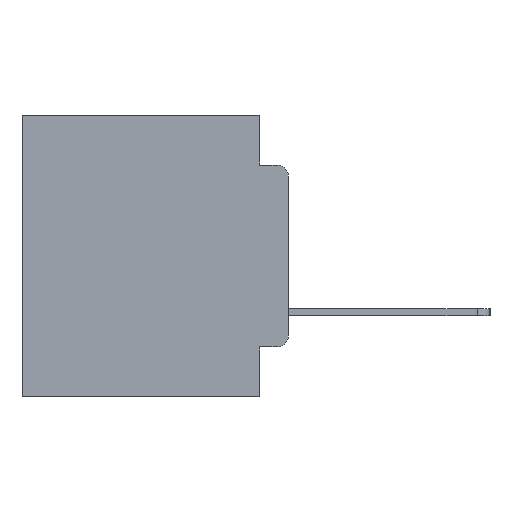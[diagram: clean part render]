
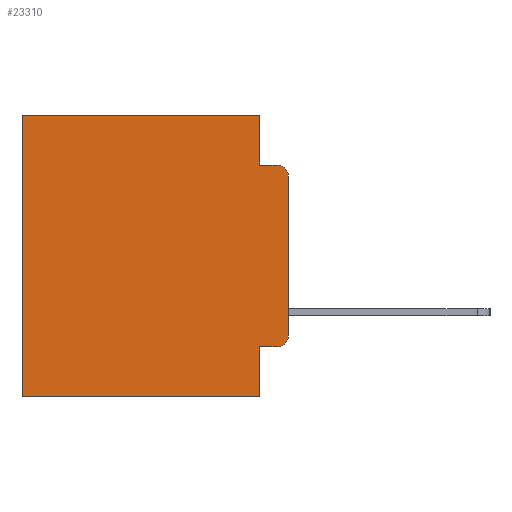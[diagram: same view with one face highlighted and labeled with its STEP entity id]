
A CAD part, left-side view. The second image highlights one B-rep face of the part: STEP entity #23310.
In plain terms, the highlighted planar face has unit normal (-1, 0, 0).
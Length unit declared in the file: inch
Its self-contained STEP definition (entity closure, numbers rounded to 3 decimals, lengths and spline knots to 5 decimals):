
#515 = VERTEX_POINT ( 'NONE', #2719 ) ;
#651 = CARTESIAN_POINT ( 'NONE',  ( 0.298, 0., -0.5 ) ) ;
#841 = EDGE_CURVE ( 'NONE', #9503, #11360, #6583, .T. ) ;
#1132 = CARTESIAN_POINT ( 'NONE',  ( 0.298, 0., -0.1085 ) ) ;
#2231 = ORIENTED_EDGE ( 'NONE', *, *, #3805, .T. ) ;
#2338 = EDGE_CURVE ( 'NONE', #9503, #2474, #14834, .T. ) ;
#2396 = CARTESIAN_POINT ( 'NONE',  ( 0.298, 0.473, 0. ) ) ;
#2474 = VERTEX_POINT ( 'NONE', #25600 ) ;
#2607 = CARTESIAN_POINT ( 'NONE',  ( 0.298, 0.02, -0.4115 ) ) ;
#2719 = CARTESIAN_POINT ( 'NONE',  ( 0.298, 0., -0.3915 ) ) ;
#2882 = DIRECTION ( 'NONE',  ( 0., 1., 0. ) ) ;
#3184 = VECTOR ( 'NONE', #17346, 39.37008 ) ;
#3805 = EDGE_CURVE ( 'NONE', #10068, #22903, #26704, .T. ) ;
#4160 = CARTESIAN_POINT ( 'NONE',  ( 0.298, 0., 0. ) ) ;
#4231 = LINE ( 'NONE', #8082, #25901 ) ;
#4337 = LINE ( 'NONE', #25617, #26009 ) ;
#5426 = AXIS2_PLACEMENT_3D ( 'NONE', #4160, #23135, #10637 ) ;
#5854 = DIRECTION ( 'NONE',  ( 0., -1., 0. ) ) ;
#6113 = DIRECTION ( 'NONE',  ( 0., 0., -1. ) ) ;
#6281 = AXIS2_PLACEMENT_3D ( 'NONE', #19932, #7382, #22053 ) ;
#6313 = DIRECTION ( 'NONE',  ( 0., 0., -1. ) ) ;
#6583 = LINE ( 'NONE', #18797, #17134 ) ;
#6631 = CARTESIAN_POINT ( 'NONE',  ( 0.298, 0.051, -0.4115 ) ) ;
#6739 = EDGE_CURVE ( 'NONE', #25268, #25956, #12794, .T. ) ;
#7143 = VECTOR ( 'NONE', #24099, 39.37008 ) ;
#7382 = DIRECTION ( 'NONE',  ( -1., 0., 0. ) ) ;
#7748 = FACE_OUTER_BOUND ( 'NONE', #19220, .T. ) ;
#8082 = CARTESIAN_POINT ( 'NONE',  ( 0.298, 0., 0. ) ) ;
#8190 = EDGE_CURVE ( 'NONE', #25956, #24409, #4337, .T. ) ;
#8377 = ORIENTED_EDGE ( 'NONE', *, *, #9602, .T. ) ;
#9370 = ORIENTED_EDGE ( 'NONE', *, *, #841, .T. ) ;
#9503 = VERTEX_POINT ( 'NONE', #6631 ) ;
#9602 = EDGE_CURVE ( 'NONE', #19210, #24409, #12282, .T. ) ;
#10068 = VERTEX_POINT ( 'NONE', #2396 ) ;
#10109 = VECTOR ( 'NONE', #6113, 39.37008 ) ;
#10637 = DIRECTION ( 'NONE',  ( 0., 0., -1. ) ) ;
#11360 = VERTEX_POINT ( 'NONE', #2607 ) ;
#12282 = CIRCLE ( 'NONE', #6281, 0.02 ) ;
#12420 = EDGE_CURVE ( 'NONE', #19210, #515, #4231, .T. ) ;
#12647 = EDGE_CURVE ( 'NONE', #25268, #10068, #20061, .T. ) ;
#12650 = CARTESIAN_POINT ( 'NONE',  ( 0.298, 0.02, -0.3915 ) ) ;
#12675 = PLANE ( 'NONE',  #5426 ) ;
#12794 = LINE ( 'NONE', #22020, #7143 ) ;
#13660 = ORIENTED_EDGE ( 'NONE', *, *, #2338, .F. ) ;
#14770 = DIRECTION ( 'NONE',  ( 0., 0., -1. ) ) ;
#14834 = LINE ( 'NONE', #15004, #19034 ) ;
#15004 = CARTESIAN_POINT ( 'NONE',  ( 0.298, 0.051, 0. ) ) ;
#15262 = CARTESIAN_POINT ( 'NONE',  ( 0.298, 0., 0. ) ) ;
#15452 = CARTESIAN_POINT ( 'NONE',  ( 0.298, 0.473, -0.5 ) ) ;
#15798 = CARTESIAN_POINT ( 'NONE',  ( 0.298, 0.051, -0.0885 ) ) ;
#16183 = DIRECTION ( 'NONE',  ( 0., -1., 0. ) ) ;
#16511 = EDGE_CURVE ( 'NONE', #2474, #22903, #26353, .T. ) ;
#16595 = ORIENTED_EDGE ( 'NONE', *, *, #8190, .F. ) ;
#16808 = CARTESIAN_POINT ( 'NONE',  ( 0.298, 0.473, 0. ) ) ;
#17134 = VECTOR ( 'NONE', #5854, 39.37008 ) ;
#17346 = DIRECTION ( 'NONE',  ( 0., 1., 0. ) ) ;
#17883 = ORIENTED_EDGE ( 'NONE', *, *, #12647, .T. ) ;
#18680 = AXIS2_PLACEMENT_3D ( 'NONE', #12650, #27131, #14770 ) ;
#18797 = CARTESIAN_POINT ( 'NONE',  ( 0.298, 0.051, -0.4115 ) ) ;
#19034 = VECTOR ( 'NONE', #6313, 39.37008 ) ;
#19167 = ORIENTED_EDGE ( 'NONE', *, *, #16511, .F. ) ;
#19210 = VERTEX_POINT ( 'NONE', #1132 ) ;
#19220 = EDGE_LOOP ( 'NONE', ( #26283, #8377, #16595, #23405, #17883, #2231, #19167, #13660, #9370, #20463 ) ) ;
#19316 = CARTESIAN_POINT ( 'NONE',  ( 0.298, 0.051, 0. ) ) ;
#19932 = CARTESIAN_POINT ( 'NONE',  ( 0.298, 0.02, -0.1085 ) ) ;
#20061 = LINE ( 'NONE', #15262, #3184 ) ;
#20463 = ORIENTED_EDGE ( 'NONE', *, *, #26836, .T. ) ;
#20631 = CARTESIAN_POINT ( 'NONE',  ( 0.298, 0.02, -0.0885 ) ) ;
#20766 = CIRCLE ( 'NONE', #18680, 0.02 ) ;
#22020 = CARTESIAN_POINT ( 'NONE',  ( 0.298, 0.051, 0. ) ) ;
#22053 = DIRECTION ( 'NONE',  ( 0., 0., -1. ) ) ;
#22719 = DIRECTION ( 'NONE',  ( 0., 0., -1. ) ) ;
#22903 = VERTEX_POINT ( 'NONE', #15452 ) ;
#23135 = DIRECTION ( 'NONE',  ( 1., 0., 0. ) ) ;
#23310 = ADVANCED_FACE ( 'NONE', ( #7748 ), #12675, .F. ) ;
#23405 = ORIENTED_EDGE ( 'NONE', *, *, #6739, .F. ) ;
#24099 = DIRECTION ( 'NONE',  ( 0., 0., -1. ) ) ;
#24409 = VERTEX_POINT ( 'NONE', #20631 ) ;
#25268 = VERTEX_POINT ( 'NONE', #19316 ) ;
#25600 = CARTESIAN_POINT ( 'NONE',  ( 0.298, 0.051, -0.5 ) ) ;
#25617 = CARTESIAN_POINT ( 'NONE',  ( 0.298, 0.051, -0.0885 ) ) ;
#25711 = VECTOR ( 'NONE', #2882, 39.37008 ) ;
#25901 = VECTOR ( 'NONE', #22719, 39.37008 ) ;
#25956 = VERTEX_POINT ( 'NONE', #15798 ) ;
#26009 = VECTOR ( 'NONE', #16183, 39.37008 ) ;
#26283 = ORIENTED_EDGE ( 'NONE', *, *, #12420, .F. ) ;
#26353 = LINE ( 'NONE', #651, #25711 ) ;
#26704 = LINE ( 'NONE', #16808, #10109 ) ;
#26836 = EDGE_CURVE ( 'NONE', #11360, #515, #20766, .T. ) ;
#27131 = DIRECTION ( 'NONE',  ( -1., 0., 0. ) ) ;
